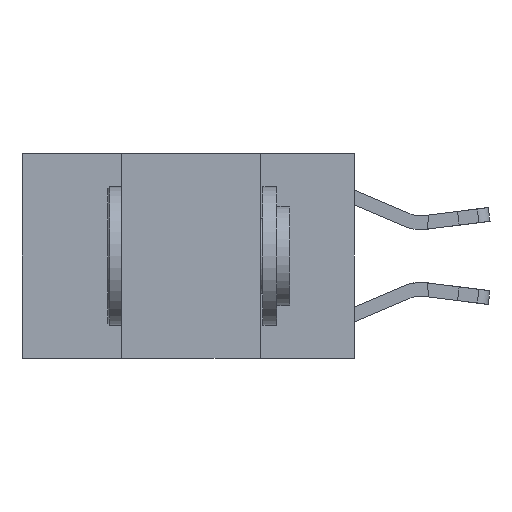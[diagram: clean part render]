
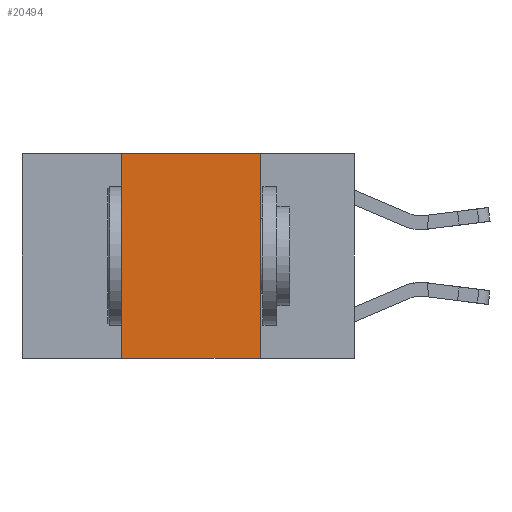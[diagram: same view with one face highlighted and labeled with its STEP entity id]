
A CAD part, left-side view. The second image highlights one B-rep face of the part: STEP entity #20494.
In plain terms, the highlighted planar face has unit normal (-1, 0, 0).
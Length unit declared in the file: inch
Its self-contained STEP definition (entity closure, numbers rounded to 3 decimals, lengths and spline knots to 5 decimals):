
#667 = ORIENTED_EDGE ( 'NONE', *, *, #19920, .F. ) ;
#686 = AXIS2_PLACEMENT_3D ( 'NONE', #8547, #12599, #1997 ) ;
#1518 = PLANE ( 'NONE',  #686 ) ;
#1997 = DIRECTION ( 'NONE',  ( 0., 0., -1. ) ) ;
#2752 = ORIENTED_EDGE ( 'NONE', *, *, #4756, .F. ) ;
#4756 = EDGE_CURVE ( 'NONE', #22445, #17573, #10164, .T. ) ;
#4917 = LINE ( 'NONE', #10220, #21684 ) ;
#5110 = EDGE_LOOP ( 'NONE', ( #667, #2752, #11273, #14897 ) ) ;
#5875 = VERTEX_POINT ( 'NONE', #14985 ) ;
#8131 = VECTOR ( 'NONE', #13928, 39.37008 ) ;
#8455 = VERTEX_POINT ( 'NONE', #10544 ) ;
#8547 = CARTESIAN_POINT ( 'NONE',  ( 0., 0.6, 0. ) ) ;
#8753 = EDGE_CURVE ( 'NONE', #5875, #8455, #13268, .T. ) ;
#10164 = LINE ( 'NONE', #15573, #8131 ) ;
#10220 = CARTESIAN_POINT ( 'NONE',  ( 0., 0.17, 0. ) ) ;
#10544 = CARTESIAN_POINT ( 'NONE',  ( 0., 0.17, -0.37 ) ) ;
#11273 = ORIENTED_EDGE ( 'NONE', *, *, #21454, .F. ) ;
#11561 = DIRECTION ( 'NONE',  ( 0., -1., 0. ) ) ;
#11943 = DIRECTION ( 'NONE',  ( 0., 0., -1. ) ) ;
#12295 = CARTESIAN_POINT ( 'NONE',  ( 0., 0.17, 0. ) ) ;
#12430 = LINE ( 'NONE', #17498, #18021 ) ;
#12599 = DIRECTION ( 'NONE',  ( 1., 0., 0. ) ) ;
#13268 = LINE ( 'NONE', #18690, #15908 ) ;
#13888 = CARTESIAN_POINT ( 'NONE',  ( 0., 0.42, 0. ) ) ;
#13928 = DIRECTION ( 'NONE',  ( 0., -1., 0. ) ) ;
#14018 = DIRECTION ( 'NONE',  ( 0., 0., 1. ) ) ;
#14897 = ORIENTED_EDGE ( 'NONE', *, *, #8753, .T. ) ;
#14985 = CARTESIAN_POINT ( 'NONE',  ( 0., 0.42, -0.37 ) ) ;
#15573 = CARTESIAN_POINT ( 'NONE',  ( 0., 0.6, 0. ) ) ;
#15908 = VECTOR ( 'NONE', #11561, 39.37008 ) ;
#17498 = CARTESIAN_POINT ( 'NONE',  ( 0., 0.42, 0. ) ) ;
#17573 = VERTEX_POINT ( 'NONE', #12295 ) ;
#18021 = VECTOR ( 'NONE', #14018, 39.37008 ) ;
#18690 = CARTESIAN_POINT ( 'NONE',  ( 0., 0.6, -0.37 ) ) ;
#19920 = EDGE_CURVE ( 'NONE', #17573, #8455, #4917, .T. ) ;
#20494 = ADVANCED_FACE ( 'NONE', ( #20753 ), #1518, .F. ) ;
#20753 = FACE_OUTER_BOUND ( 'NONE', #5110, .T. ) ;
#21454 = EDGE_CURVE ( 'NONE', #5875, #22445, #12430, .T. ) ;
#21684 = VECTOR ( 'NONE', #11943, 39.37008 ) ;
#22445 = VERTEX_POINT ( 'NONE', #13888 ) ;
